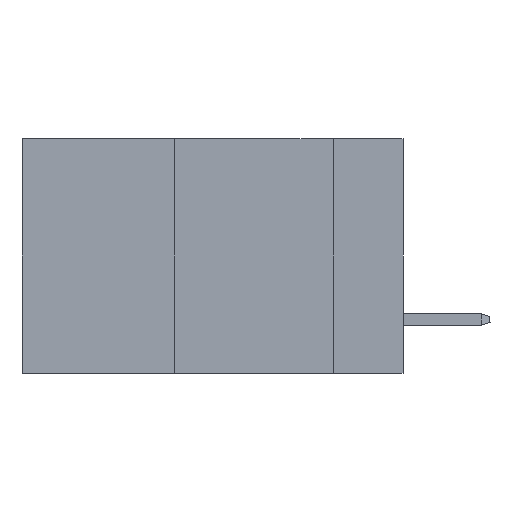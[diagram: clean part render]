
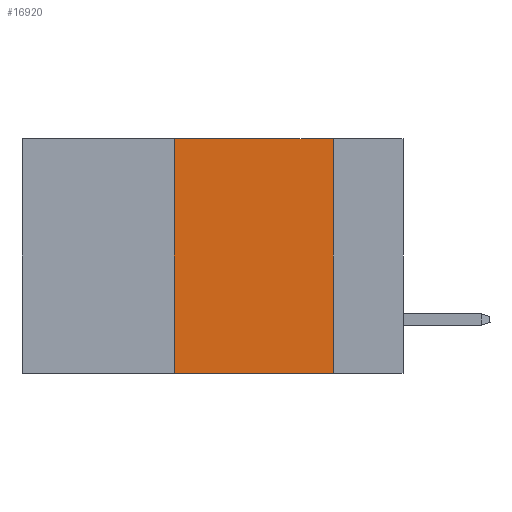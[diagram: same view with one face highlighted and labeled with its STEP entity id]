
A CAD part, left-side view. The second image highlights one B-rep face of the part: STEP entity #16920.
In plain terms, the highlighted planar face has unit normal (-1, 0, 0).
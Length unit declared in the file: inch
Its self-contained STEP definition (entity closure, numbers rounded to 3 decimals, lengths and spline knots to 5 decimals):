
#981 = VECTOR ( 'NONE', #8023, 39.37008 ) ;
#1152 = AXIS2_PLACEMENT_3D ( 'NONE', #14468, #2679, #12670 ) ;
#2106 = VERTEX_POINT ( 'NONE', #13140 ) ;
#2390 = EDGE_CURVE ( 'NONE', #6593, #7886, #13707, .T. ) ;
#2679 = DIRECTION ( 'NONE',  ( 1., 0., 0. ) ) ;
#3000 = VECTOR ( 'NONE', #12942, 39.37008 ) ;
#3390 = EDGE_CURVE ( 'NONE', #2106, #12203, #16844, .T. ) ;
#4251 = CARTESIAN_POINT ( 'NONE',  ( 0., 0.36, 0. ) ) ;
#4334 = CARTESIAN_POINT ( 'NONE',  ( 0., 0.11, 0. ) ) ;
#5764 = ORIENTED_EDGE ( 'NONE', *, *, #3390, .T. ) ;
#6593 = VERTEX_POINT ( 'NONE', #15167 ) ;
#6961 = CARTESIAN_POINT ( 'NONE',  ( 0., 0.11, 0. ) ) ;
#6974 = FACE_OUTER_BOUND ( 'NONE', #10054, .T. ) ;
#7886 = VERTEX_POINT ( 'NONE', #4334 ) ;
#7927 = CARTESIAN_POINT ( 'NONE',  ( 0., 0.6, 0. ) ) ;
#8023 = DIRECTION ( 'NONE',  ( 0., -1., 0. ) ) ;
#8555 = EDGE_CURVE ( 'NONE', #2106, #6593, #17313, .T. ) ;
#8836 = DIRECTION ( 'NONE',  ( 0., 0., 1. ) ) ;
#9730 = LINE ( 'NONE', #6961, #3000 ) ;
#10054 = EDGE_LOOP ( 'NONE', ( #17634, #15877, #17545, #5764 ) ) ;
#12203 = VERTEX_POINT ( 'NONE', #17452 ) ;
#12465 = CARTESIAN_POINT ( 'NONE',  ( 0., 0.6, -0.37 ) ) ;
#12670 = DIRECTION ( 'NONE',  ( 0., 0., -1. ) ) ;
#12942 = DIRECTION ( 'NONE',  ( 0., 0., -1. ) ) ;
#13066 = PLANE ( 'NONE',  #1152 ) ;
#13140 = CARTESIAN_POINT ( 'NONE',  ( 0., 0.36, -0.37 ) ) ;
#13707 = LINE ( 'NONE', #7927, #981 ) ;
#14468 = CARTESIAN_POINT ( 'NONE',  ( 0., 0.6, 0. ) ) ;
#15130 = DIRECTION ( 'NONE',  ( 0., -1., 0. ) ) ;
#15167 = CARTESIAN_POINT ( 'NONE',  ( 0., 0.36, 0. ) ) ;
#15877 = ORIENTED_EDGE ( 'NONE', *, *, #2390, .F. ) ;
#16074 = VECTOR ( 'NONE', #8836, 39.37008 ) ;
#16733 = EDGE_CURVE ( 'NONE', #7886, #12203, #9730, .T. ) ;
#16844 = LINE ( 'NONE', #12465, #17170 ) ;
#16920 = ADVANCED_FACE ( 'NONE', ( #6974 ), #13066, .F. ) ;
#17170 = VECTOR ( 'NONE', #15130, 39.37008 ) ;
#17313 = LINE ( 'NONE', #4251, #16074 ) ;
#17452 = CARTESIAN_POINT ( 'NONE',  ( 0., 0.11, -0.37 ) ) ;
#17545 = ORIENTED_EDGE ( 'NONE', *, *, #8555, .F. ) ;
#17634 = ORIENTED_EDGE ( 'NONE', *, *, #16733, .F. ) ;
